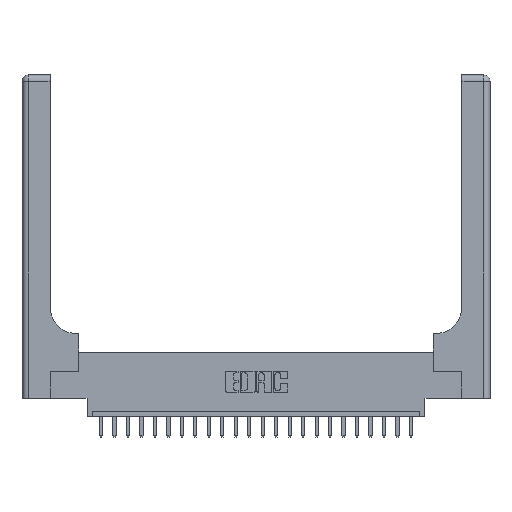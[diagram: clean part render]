
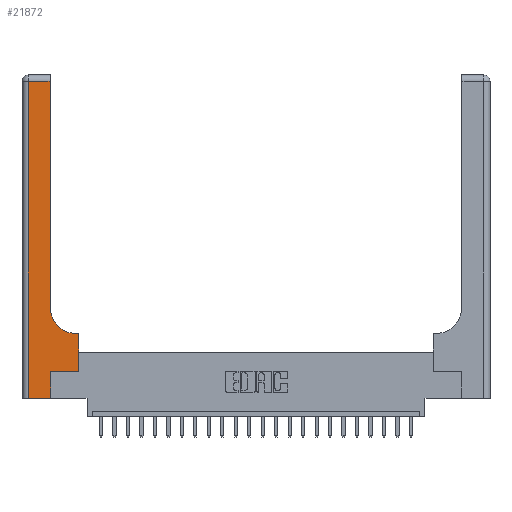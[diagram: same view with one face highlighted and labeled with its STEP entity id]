
A CAD part, top view. The second image highlights one B-rep face of the part: STEP entity #21872.
In plain terms, the highlighted planar face has unit normal (0, 0, 1).
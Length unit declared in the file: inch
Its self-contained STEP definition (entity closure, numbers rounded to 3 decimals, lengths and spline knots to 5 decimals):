
#1137 = LINE ( 'NONE', #18072, #3610 ) ;
#1711 = CARTESIAN_POINT ( 'NONE',  ( 0.265, 0., 0.37 ) ) ;
#1984 = CARTESIAN_POINT ( 'NONE',  ( 0., 0., 0.37 ) ) ;
#2094 = ORIENTED_EDGE ( 'NONE', *, *, #19425, .T. ) ;
#2723 = CARTESIAN_POINT ( 'NONE',  ( 0.06, 3., 0.37 ) ) ;
#3573 = VERTEX_POINT ( 'NONE', #14924 ) ;
#3610 = VECTOR ( 'NONE', #14883, 39.37008 ) ;
#3748 = EDGE_CURVE ( 'NONE', #19843, #8914, #5047, .T. ) ;
#3880 = VECTOR ( 'NONE', #22718, 39.37008 ) ;
#3888 = ORIENTED_EDGE ( 'NONE', *, *, #13519, .T. ) ;
#4583 = ORIENTED_EDGE ( 'NONE', *, *, #19840, .T. ) ;
#4879 = AXIS2_PLACEMENT_3D ( 'NONE', #5612, #7380, #9130 ) ;
#5047 = LINE ( 'NONE', #10053, #5590 ) ;
#5590 = VECTOR ( 'NONE', #17034, 39.37008 ) ;
#5612 = CARTESIAN_POINT ( 'NONE',  ( 0.51, 0.85, 0.37 ) ) ;
#6067 = CARTESIAN_POINT ( 'NONE',  ( 0.06, 0., 0.37 ) ) ;
#6107 = ORIENTED_EDGE ( 'NONE', *, *, #11892, .T. ) ;
#6224 = DIRECTION ( 'NONE',  ( 0., -1., 0. ) ) ;
#6366 = CARTESIAN_POINT ( 'NONE',  ( 0.528, 0.6, 0.37 ) ) ;
#6464 = CARTESIAN_POINT ( 'NONE',  ( 0.528, 0.25, 0.37 ) ) ;
#6534 = CARTESIAN_POINT ( 'NONE',  ( 0.528, 0.25, 0.37 ) ) ;
#6553 = VERTEX_POINT ( 'NONE', #6067 ) ;
#7380 = DIRECTION ( 'NONE',  ( 0., 0., -1. ) ) ;
#8005 = ORIENTED_EDGE ( 'NONE', *, *, #19288, .T. ) ;
#8442 = FACE_OUTER_BOUND ( 'NONE', #17396, .T. ) ;
#8637 = DIRECTION ( 'NONE',  ( -1., 0., 0. ) ) ;
#8914 = VERTEX_POINT ( 'NONE', #10959 ) ;
#9130 = DIRECTION ( 'NONE',  ( 1., 0., 0. ) ) ;
#9406 = AXIS2_PLACEMENT_3D ( 'NONE', #21096, #14111, #8637 ) ;
#10053 = CARTESIAN_POINT ( 'NONE',  ( 0., 2.94, 0.37 ) ) ;
#10160 = CARTESIAN_POINT ( 'NONE',  ( 0.26, 0.85, 0.37 ) ) ;
#10574 = DIRECTION ( 'NONE',  ( 1., 0., 0. ) ) ;
#10959 = CARTESIAN_POINT ( 'NONE',  ( 0.06, 2.94, 0.37 ) ) ;
#11094 = LINE ( 'NONE', #2723, #15241 ) ;
#11314 = LINE ( 'NONE', #6534, #18234 ) ;
#11486 = DIRECTION ( 'NONE',  ( 1., 0., 0. ) ) ;
#11841 = CARTESIAN_POINT ( 'NONE',  ( 0.26, 0.6, 0.37 ) ) ;
#11892 = EDGE_CURVE ( 'NONE', #12593, #3573, #22484, .T. ) ;
#11948 = VERTEX_POINT ( 'NONE', #1711 ) ;
#12544 = LINE ( 'NONE', #1984, #21592 ) ;
#12593 = VERTEX_POINT ( 'NONE', #6366 ) ;
#12651 = VERTEX_POINT ( 'NONE', #10160 ) ;
#12707 = ORIENTED_EDGE ( 'NONE', *, *, #22634, .T. ) ;
#13321 = ORIENTED_EDGE ( 'NONE', *, *, #14573, .T. ) ;
#13519 = EDGE_CURVE ( 'NONE', #6553, #11948, #12544, .T. ) ;
#13921 = DIRECTION ( 'NONE',  ( -1., 0., 0. ) ) ;
#14111 = DIRECTION ( 'NONE',  ( 0., 0., -1. ) ) ;
#14573 = EDGE_CURVE ( 'NONE', #8914, #6553, #11094, .T. ) ;
#14883 = DIRECTION ( 'NONE',  ( 0., 1., 0. ) ) ;
#14924 = CARTESIAN_POINT ( 'NONE',  ( 0.51, 0.6, 0.37 ) ) ;
#15034 = CARTESIAN_POINT ( 'NONE',  ( 0.265, 0.25, 0.37 ) ) ;
#15241 = VECTOR ( 'NONE', #6224, 39.37008 ) ;
#15266 = CARTESIAN_POINT ( 'NONE',  ( 0.265, 0.25, 0.37 ) ) ;
#15706 = CARTESIAN_POINT ( 'NONE',  ( 0.26, 2.94, 0.37 ) ) ;
#16065 = LINE ( 'NONE', #15034, #19333 ) ;
#16751 = EDGE_CURVE ( 'NONE', #11948, #22370, #1137, .T. ) ;
#16767 = VECTOR ( 'NONE', #13921, 39.37008 ) ;
#17034 = DIRECTION ( 'NONE',  ( -1., 0., 0. ) ) ;
#17396 = EDGE_LOOP ( 'NONE', ( #4583, #18201, #13321, #3888, #18546, #8005, #2094, #6107, #12707 ) ) ;
#18072 = CARTESIAN_POINT ( 'NONE',  ( 0.265, 0., 0.37 ) ) ;
#18201 = ORIENTED_EDGE ( 'NONE', *, *, #3748, .T. ) ;
#18234 = VECTOR ( 'NONE', #20630, 39.37008 ) ;
#18491 = LINE ( 'NONE', #20965, #3880 ) ;
#18546 = ORIENTED_EDGE ( 'NONE', *, *, #16751, .T. ) ;
#19288 = EDGE_CURVE ( 'NONE', #22370, #22289, #16065, .T. ) ;
#19333 = VECTOR ( 'NONE', #11486, 39.37008 ) ;
#19425 = EDGE_CURVE ( 'NONE', #22289, #12593, #11314, .T. ) ;
#19840 = EDGE_CURVE ( 'NONE', #12651, #19843, #18491, .T. ) ;
#19843 = VERTEX_POINT ( 'NONE', #15706 ) ;
#20630 = DIRECTION ( 'NONE',  ( 0., 1., 0. ) ) ;
#20965 = CARTESIAN_POINT ( 'NONE',  ( 0.26, 3., 0.37 ) ) ;
#21096 = CARTESIAN_POINT ( 'NONE',  ( 0., 3., 0.37 ) ) ;
#21592 = VECTOR ( 'NONE', #10574, 39.37008 ) ;
#21616 = CIRCLE ( 'NONE', #4879, 0.25 ) ;
#21872 = ADVANCED_FACE ( 'NONE', ( #8442 ), #22620, .F. ) ;
#22289 = VERTEX_POINT ( 'NONE', #6464 ) ;
#22370 = VERTEX_POINT ( 'NONE', #15266 ) ;
#22484 = LINE ( 'NONE', #11841, #16767 ) ;
#22620 = PLANE ( 'NONE',  #9406 ) ;
#22634 = EDGE_CURVE ( 'NONE', #3573, #12651, #21616, .T. ) ;
#22718 = DIRECTION ( 'NONE',  ( 0., 1., 0. ) ) ;
